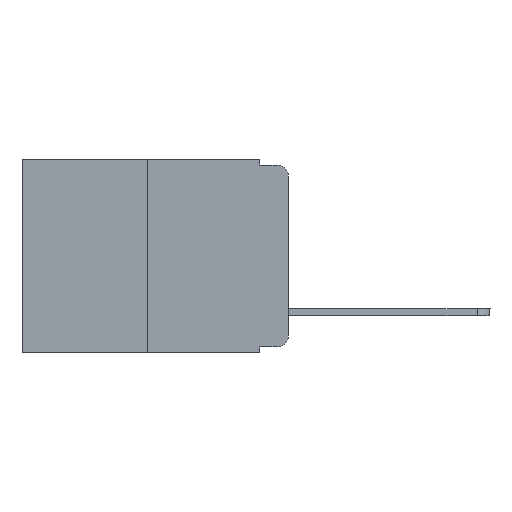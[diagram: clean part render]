
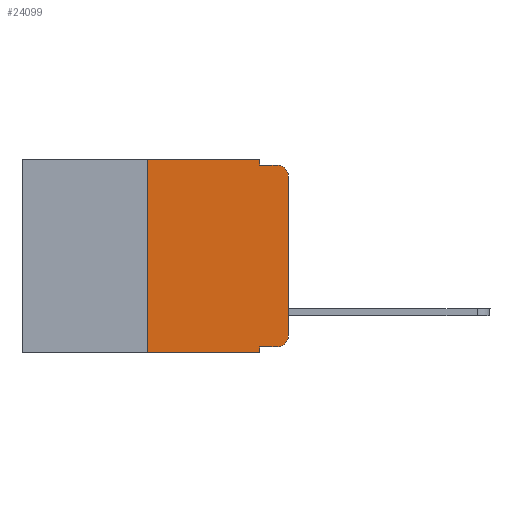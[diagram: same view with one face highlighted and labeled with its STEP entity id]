
A CAD part, left-side view. The second image highlights one B-rep face of the part: STEP entity #24099.
In plain terms, the highlighted planar face has unit normal (-1, 0, 0).
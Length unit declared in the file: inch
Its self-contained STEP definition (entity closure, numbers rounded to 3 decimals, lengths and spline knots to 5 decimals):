
#248 = EDGE_CURVE ( 'NONE', #19823, #15859, #6168, .T. ) ;
#264 = VERTEX_POINT ( 'NONE', #23128 ) ;
#359 = EDGE_CURVE ( 'NONE', #19066, #15859, #5265, .T. ) ;
#457 = CARTESIAN_POINT ( 'NONE',  ( 0., 0.051, -0.01 ) ) ;
#1108 = VERTEX_POINT ( 'NONE', #20460 ) ;
#1588 = AXIS2_PLACEMENT_3D ( 'NONE', #12263, #16186, #8570 ) ;
#1949 = DIRECTION ( 'NONE',  ( 0., -1., 0. ) ) ;
#2241 = EDGE_CURVE ( 'NONE', #19823, #25199, #23856, .T. ) ;
#2247 = CARTESIAN_POINT ( 'NONE',  ( 0., 0.02, -0.313 ) ) ;
#2415 = EDGE_CURVE ( 'NONE', #19523, #1108, #25093, .T. ) ;
#2432 = DIRECTION ( 'NONE',  ( 0., -1., 0. ) ) ;
#2500 = DIRECTION ( 'NONE',  ( 0., -1., 0. ) ) ;
#2643 = DIRECTION ( 'NONE',  ( 0., 0., -1. ) ) ;
#2948 = CARTESIAN_POINT ( 'NONE',  ( 0., 0.02, -0.01 ) ) ;
#3983 = DIRECTION ( 'NONE',  ( 0., 0., 1. ) ) ;
#4190 = LINE ( 'NONE', #21700, #8488 ) ;
#4552 = ORIENTED_EDGE ( 'NONE', *, *, #8230, .T. ) ;
#4600 = VERTEX_POINT ( 'NONE', #16203 ) ;
#4766 = VERTEX_POINT ( 'NONE', #5318 ) ;
#5265 = LINE ( 'NONE', #11985, #15698 ) ;
#5318 = CARTESIAN_POINT ( 'NONE',  ( 0., 0.02, -0.333 ) ) ;
#5972 = CARTESIAN_POINT ( 'NONE',  ( 0., 0.25, -0.343 ) ) ;
#6143 = CIRCLE ( 'NONE', #23502, 0.02 ) ;
#6168 = LINE ( 'NONE', #15256, #19660 ) ;
#6693 = ORIENTED_EDGE ( 'NONE', *, *, #17835, .T. ) ;
#6920 = LINE ( 'NONE', #21737, #8434 ) ;
#7643 = DIRECTION ( 'NONE',  ( 0., -1., 0. ) ) ;
#8230 = EDGE_CURVE ( 'NONE', #4600, #264, #4190, .T. ) ;
#8332 = ORIENTED_EDGE ( 'NONE', *, *, #19878, .F. ) ;
#8434 = VECTOR ( 'NONE', #1949, 39.37008 ) ;
#8451 = DIRECTION ( 'NONE',  ( -1., 0., 0. ) ) ;
#8488 = VECTOR ( 'NONE', #3983, 39.37008 ) ;
#8513 = CARTESIAN_POINT ( 'NONE',  ( 0., 0.051, -0.343 ) ) ;
#8570 = DIRECTION ( 'NONE',  ( 0., 0., -1. ) ) ;
#8887 = ORIENTED_EDGE ( 'NONE', *, *, #12593, .T. ) ;
#9435 = ORIENTED_EDGE ( 'NONE', *, *, #15384, .T. ) ;
#9706 = AXIS2_PLACEMENT_3D ( 'NONE', #22069, #23715, #10197 ) ;
#9942 = DIRECTION ( 'NONE',  ( 0., 0., -1. ) ) ;
#9952 = CIRCLE ( 'NONE', #1588, 0.02 ) ;
#10197 = DIRECTION ( 'NONE',  ( 0., 0., -1. ) ) ;
#10440 = FACE_OUTER_BOUND ( 'NONE', #17631, .T. ) ;
#11277 = CARTESIAN_POINT ( 'NONE',  ( 0., 0.051, -0.333 ) ) ;
#11985 = CARTESIAN_POINT ( 'NONE',  ( 0., 0.051, 0. ) ) ;
#12210 = DIRECTION ( 'NONE',  ( 0., 0., 1. ) ) ;
#12263 = CARTESIAN_POINT ( 'NONE',  ( 0., 0.02, -0.03 ) ) ;
#12323 = PLANE ( 'NONE',  #9706 ) ;
#12593 = EDGE_CURVE ( 'NONE', #264, #15053, #9952, .T. ) ;
#13760 = ORIENTED_EDGE ( 'NONE', *, *, #248, .T. ) ;
#13763 = VECTOR ( 'NONE', #2500, 39.37008 ) ;
#14165 = LINE ( 'NONE', #21824, #20268 ) ;
#14421 = CARTESIAN_POINT ( 'NONE',  ( 0., 0.051, 0. ) ) ;
#14675 = EDGE_CURVE ( 'NONE', #25199, #19523, #14165, .T. ) ;
#15053 = VERTEX_POINT ( 'NONE', #2948 ) ;
#15256 = CARTESIAN_POINT ( 'NONE',  ( 0., 0.473, -0.343 ) ) ;
#15384 = EDGE_CURVE ( 'NONE', #4766, #4600, #6143, .T. ) ;
#15698 = VECTOR ( 'NONE', #9942, 39.37008 ) ;
#15859 = VERTEX_POINT ( 'NONE', #8513 ) ;
#15876 = LINE ( 'NONE', #457, #13763 ) ;
#15891 = VECTOR ( 'NONE', #12210, 39.37008 ) ;
#16186 = DIRECTION ( 'NONE',  ( -1., 0., 0. ) ) ;
#16203 = CARTESIAN_POINT ( 'NONE',  ( 0., 0., -0.313 ) ) ;
#17631 = EDGE_LOOP ( 'NONE', ( #4552, #8887, #8332, #18900, #19390, #21850, #13760, #22109, #6693, #9435 ) ) ;
#17633 = CARTESIAN_POINT ( 'NONE',  ( 0., 0.25, 0. ) ) ;
#17769 = CARTESIAN_POINT ( 'NONE',  ( 0., 0.25, 0. ) ) ;
#17835 = EDGE_CURVE ( 'NONE', #19066, #4766, #6920, .T. ) ;
#18201 = DIRECTION ( 'NONE',  ( 0., 0., -1. ) ) ;
#18900 = ORIENTED_EDGE ( 'NONE', *, *, #2415, .F. ) ;
#19066 = VERTEX_POINT ( 'NONE', #11277 ) ;
#19390 = ORIENTED_EDGE ( 'NONE', *, *, #14675, .F. ) ;
#19523 = VERTEX_POINT ( 'NONE', #22696 ) ;
#19660 = VECTOR ( 'NONE', #7643, 39.37008 ) ;
#19823 = VERTEX_POINT ( 'NONE', #5972 ) ;
#19878 = EDGE_CURVE ( 'NONE', #1108, #15053, #15876, .T. ) ;
#20268 = VECTOR ( 'NONE', #2432, 39.37008 ) ;
#20460 = CARTESIAN_POINT ( 'NONE',  ( 0., 0.051, -0.01 ) ) ;
#21101 = VECTOR ( 'NONE', #2643, 39.37008 ) ;
#21700 = CARTESIAN_POINT ( 'NONE',  ( 0., 0., 0. ) ) ;
#21737 = CARTESIAN_POINT ( 'NONE',  ( 0., 0.051, -0.333 ) ) ;
#21824 = CARTESIAN_POINT ( 'NONE',  ( 0., 0.473, 0. ) ) ;
#21850 = ORIENTED_EDGE ( 'NONE', *, *, #2241, .F. ) ;
#22069 = CARTESIAN_POINT ( 'NONE',  ( 0., 0.473, 0. ) ) ;
#22109 = ORIENTED_EDGE ( 'NONE', *, *, #359, .F. ) ;
#22696 = CARTESIAN_POINT ( 'NONE',  ( 0., 0.051, 0. ) ) ;
#23128 = CARTESIAN_POINT ( 'NONE',  ( 0., 0., -0.03 ) ) ;
#23502 = AXIS2_PLACEMENT_3D ( 'NONE', #2247, #8451, #18201 ) ;
#23715 = DIRECTION ( 'NONE',  ( 1., 0., 0. ) ) ;
#23856 = LINE ( 'NONE', #17769, #15891 ) ;
#24099 = ADVANCED_FACE ( 'NONE', ( #10440 ), #12323, .F. ) ;
#25093 = LINE ( 'NONE', #14421, #21101 ) ;
#25199 = VERTEX_POINT ( 'NONE', #17633 ) ;
